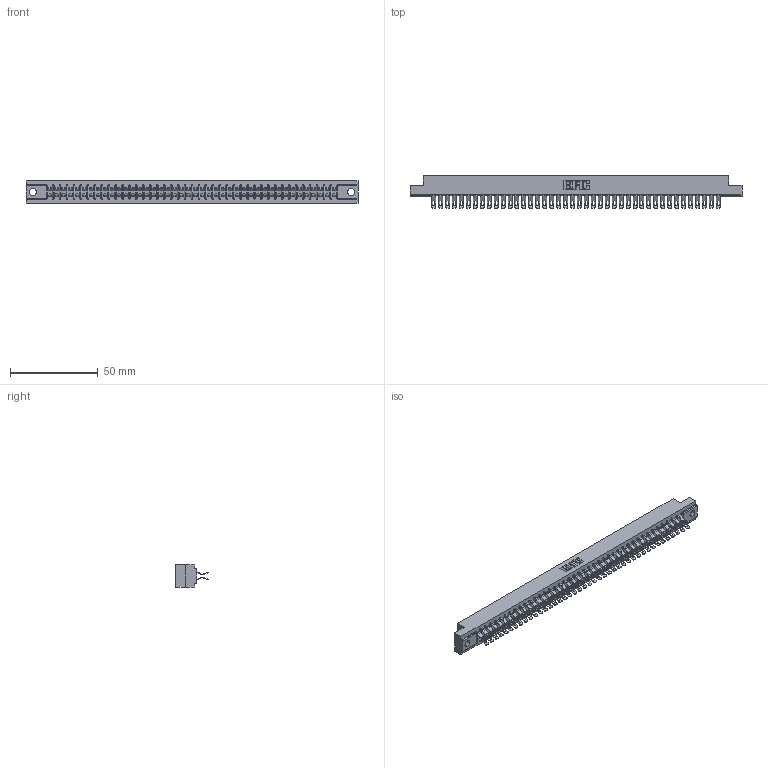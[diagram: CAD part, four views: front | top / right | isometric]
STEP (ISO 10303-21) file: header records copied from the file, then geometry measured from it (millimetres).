
FILE_DESCRIPTION (( 'STEP AP203' ), '1' );
FILE_NAME ('357-084-455-204.STEP', '2020-10-04T07:53:23', ( '' ), ( '' ), 'SwSTEP 2.0', 'SolidWorks 2020', '' );
FILE_SCHEMA (( 'CONFIG_CONTROL_DESIGN' ));
Length unit declared in the file: inch
Products named in the file (3): 307-290-001_555; 307 Part_.156 Dia Mounting Holes; 357-084-455-204
Assembly tree (85 placements, depth 2):
  357-084-455-204
    307 Part_.156 Dia Mounting Holes
    307-290-001_555  x84
Bounding box: 189.43 x 18.75 x 12.7 mm (x, y, z)
Volume: 20288.3 mm3; surface area: 26046.4 mm2
Topology: 85 solids, 85 shells, 5299 faces, 15563 edges, 10146 vertices
Faces by surface type: plane 2940, cylinder 2273, sphere 86
Entity records: 38305 total; most frequent: CARTESIAN_POINT 6276, ORIENTED_EDGE 6220, DIRECTION 6146, EDGE_CURVE 3110, LINE 2382, VECTOR 2382, VERTEX_POINT 2012, AXIS2_PLACEMENT_3D 1882
